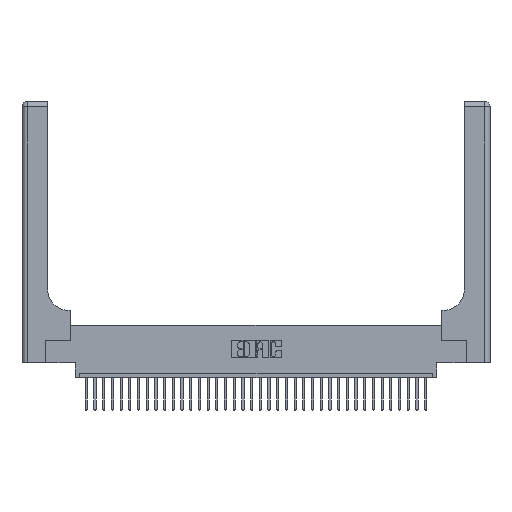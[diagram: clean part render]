
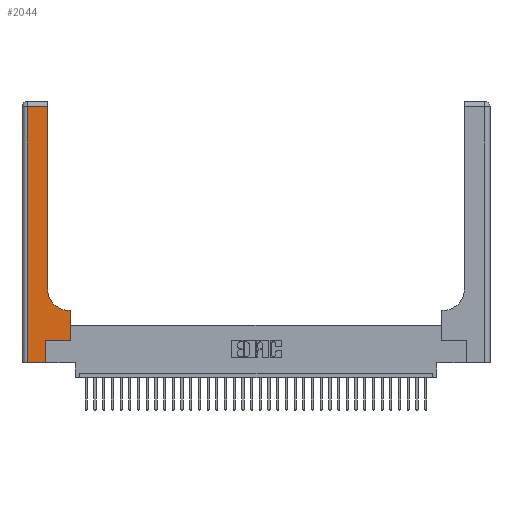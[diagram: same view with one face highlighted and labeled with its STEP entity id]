
A CAD part, top view. The second image highlights one B-rep face of the part: STEP entity #2044.
In plain terms, the highlighted planar face has unit normal (0, 0, 1).
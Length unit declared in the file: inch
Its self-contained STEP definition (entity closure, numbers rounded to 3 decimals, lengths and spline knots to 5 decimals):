
#178 = LINE ( 'NONE', #17822, #10541 ) ;
#568 = LINE ( 'NONE', #30067, #16142 ) ;
#1159 = ORIENTED_EDGE ( 'NONE', *, *, #5594, .T. ) ;
#1888 = ORIENTED_EDGE ( 'NONE', *, *, #7877, .T. ) ;
#1890 = VECTOR ( 'NONE', #34420, 39.37008 ) ;
#2034 = EDGE_CURVE ( 'NONE', #16632, #12346, #25597, .T. ) ;
#2044 = ADVANCED_FACE ( 'NONE', ( #34658 ), #4692, .F. ) ;
#2316 = DIRECTION ( 'NONE',  ( 0., 1., 0. ) ) ;
#2618 = CARTESIAN_POINT ( 'NONE',  ( 0.5415, 0.6, 0.37 ) ) ;
#3340 = CARTESIAN_POINT ( 'NONE',  ( 0.2915, 2.94, 0.37 ) ) ;
#4629 = LINE ( 'NONE', #13180, #18836 ) ;
#4692 = PLANE ( 'NONE',  #10396 ) ;
#4841 = AXIS2_PLACEMENT_3D ( 'NONE', #12301, #31591, #15115 ) ;
#5017 = LINE ( 'NONE', #9541, #26146 ) ;
#5594 = EDGE_CURVE ( 'NONE', #24087, #13980, #14092, .T. ) ;
#6722 = ORIENTED_EDGE ( 'NONE', *, *, #10961, .T. ) ;
#7468 = DIRECTION ( 'NONE',  ( 0., 0., -1. ) ) ;
#7877 = EDGE_CURVE ( 'NONE', #17174, #24087, #5017, .T. ) ;
#9541 = CARTESIAN_POINT ( 'NONE',  ( 0.06, 3., 0.37 ) ) ;
#10308 = CARTESIAN_POINT ( 'NONE',  ( 0.06, 2.94, 0.37 ) ) ;
#10315 = EDGE_CURVE ( 'NONE', #24058, #23543, #178, .T. ) ;
#10396 = AXIS2_PLACEMENT_3D ( 'NONE', #29134, #7468, #35055 ) ;
#10541 = VECTOR ( 'NONE', #19965, 39.37008 ) ;
#10961 = EDGE_CURVE ( 'NONE', #22719, #17174, #25185, .T. ) ;
#11623 = CARTESIAN_POINT ( 'NONE',  ( 0.269, 0.25, 0.37 ) ) ;
#11943 = DIRECTION ( 'NONE',  ( 0., 1., 0. ) ) ;
#11998 = CARTESIAN_POINT ( 'NONE',  ( 0., 2.94, 0.37 ) ) ;
#12301 = CARTESIAN_POINT ( 'NONE',  ( 0.5415, 0.85, 0.37 ) ) ;
#12346 = VERTEX_POINT ( 'NONE', #20525 ) ;
#12442 = LINE ( 'NONE', #24055, #23675 ) ;
#12639 = EDGE_CURVE ( 'NONE', #23543, #13767, #31108, .T. ) ;
#13180 = CARTESIAN_POINT ( 'NONE',  ( 0.5585, 0.25, 0.37 ) ) ;
#13578 = ORIENTED_EDGE ( 'NONE', *, *, #23756, .T. ) ;
#13767 = VERTEX_POINT ( 'NONE', #23194 ) ;
#13980 = VERTEX_POINT ( 'NONE', #19857 ) ;
#14092 = LINE ( 'NONE', #35071, #25735 ) ;
#15115 = DIRECTION ( 'NONE',  ( 1., 0., 0. ) ) ;
#16142 = VECTOR ( 'NONE', #29943, 39.37008 ) ;
#16632 = VERTEX_POINT ( 'NONE', #11623 ) ;
#17174 = VERTEX_POINT ( 'NONE', #10308 ) ;
#17822 = CARTESIAN_POINT ( 'NONE',  ( 0.2915, 0.6, 0.37 ) ) ;
#18801 = EDGE_LOOP ( 'NONE', ( #13578, #6722, #1888, #1159, #34491, #33970, #29954, #22484, #34468 ) ) ;
#18836 = VECTOR ( 'NONE', #11943, 39.37008 ) ;
#19119 = VECTOR ( 'NONE', #34941, 39.37008 ) ;
#19857 = CARTESIAN_POINT ( 'NONE',  ( 0.269, 0., 0.37 ) ) ;
#19965 = DIRECTION ( 'NONE',  ( -1., 0., 0. ) ) ;
#20525 = CARTESIAN_POINT ( 'NONE',  ( 0.5585, 0.25, 0.37 ) ) ;
#21489 = EDGE_CURVE ( 'NONE', #12346, #24058, #4629, .T. ) ;
#22484 = ORIENTED_EDGE ( 'NONE', *, *, #10315, .T. ) ;
#22719 = VERTEX_POINT ( 'NONE', #3340 ) ;
#23194 = CARTESIAN_POINT ( 'NONE',  ( 0.2915, 0.85, 0.37 ) ) ;
#23543 = VERTEX_POINT ( 'NONE', #2618 ) ;
#23675 = VECTOR ( 'NONE', #2316, 39.37008 ) ;
#23756 = EDGE_CURVE ( 'NONE', #13767, #22719, #568, .T. ) ;
#24055 = CARTESIAN_POINT ( 'NONE',  ( 0.269, 0., 0.37 ) ) ;
#24058 = VERTEX_POINT ( 'NONE', #34412 ) ;
#24087 = VERTEX_POINT ( 'NONE', #26219 ) ;
#25185 = LINE ( 'NONE', #11998, #1890 ) ;
#25597 = LINE ( 'NONE', #32277, #19119 ) ;
#25735 = VECTOR ( 'NONE', #34950, 39.37008 ) ;
#26146 = VECTOR ( 'NONE', #26160, 39.37008 ) ;
#26160 = DIRECTION ( 'NONE',  ( 0., -1., 0. ) ) ;
#26219 = CARTESIAN_POINT ( 'NONE',  ( 0.06, 0., 0.37 ) ) ;
#26297 = EDGE_CURVE ( 'NONE', #13980, #16632, #12442, .T. ) ;
#29134 = CARTESIAN_POINT ( 'NONE',  ( 0., 3., 0.37 ) ) ;
#29943 = DIRECTION ( 'NONE',  ( 0., 1., 0. ) ) ;
#29954 = ORIENTED_EDGE ( 'NONE', *, *, #21489, .T. ) ;
#30067 = CARTESIAN_POINT ( 'NONE',  ( 0.2915, 3., 0.37 ) ) ;
#31108 = CIRCLE ( 'NONE', #4841, 0.25 ) ;
#31591 = DIRECTION ( 'NONE',  ( 0., 0., -1. ) ) ;
#32277 = CARTESIAN_POINT ( 'NONE',  ( 0.269, 0.25, 0.37 ) ) ;
#33970 = ORIENTED_EDGE ( 'NONE', *, *, #2034, .T. ) ;
#34412 = CARTESIAN_POINT ( 'NONE',  ( 0.5585, 0.6, 0.37 ) ) ;
#34420 = DIRECTION ( 'NONE',  ( -1., 0., 0. ) ) ;
#34468 = ORIENTED_EDGE ( 'NONE', *, *, #12639, .T. ) ;
#34491 = ORIENTED_EDGE ( 'NONE', *, *, #26297, .T. ) ;
#34658 = FACE_OUTER_BOUND ( 'NONE', #18801, .T. ) ;
#34941 = DIRECTION ( 'NONE',  ( 1., 0., 0. ) ) ;
#34950 = DIRECTION ( 'NONE',  ( 1., 0., 0. ) ) ;
#35055 = DIRECTION ( 'NONE',  ( -1., 0., 0. ) ) ;
#35071 = CARTESIAN_POINT ( 'NONE',  ( 0., 0., 0.37 ) ) ;
